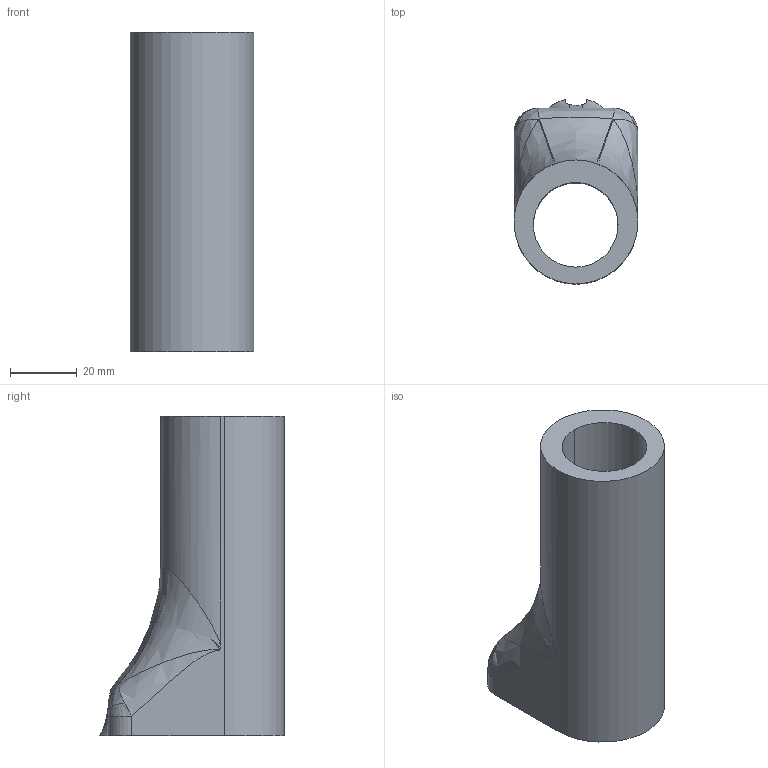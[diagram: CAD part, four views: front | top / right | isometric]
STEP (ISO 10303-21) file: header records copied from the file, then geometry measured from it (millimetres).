
FILE_DESCRIPTION (( 'STEP AP214' ), '1' );
FILE_NAME ('7.STEP', '2013-09-29T07:09:04', ( 'elpi' ), ( '' ), 'SwSTEP 2.0', 'SolidWorks 2013', '' );
FILE_SCHEMA (( 'AUTOMOTIVE_DESIGN' ));
Length unit declared in the file: millimetre
Products named in the file (1): 7
Bounding box: 37.13 x 55.42 x 95.81 mm (x, y, z)
Volume: 71647.3 mm3; surface area: 21877.9 mm2
Topology: 1 solids, 1 shells, 29 faces, 75 edges, 48 vertices
Faces by surface type: bspline 12, cylinder 9, plane 6, torus 2
Entity records: 2312 total; most frequent: CARTESIAN_POINT 1676, ORIENTED_EDGE 150, DIRECTION 93, EDGE_CURVE 75, VERTEX_POINT 48, AXIS2_PLACEMENT_3D 37, EDGE_LOOP 31, B_SPLINE_CURVE_WITH_KNOTS 30
